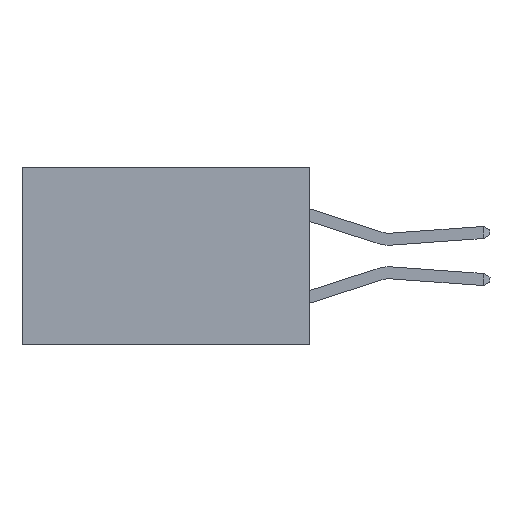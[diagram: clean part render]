
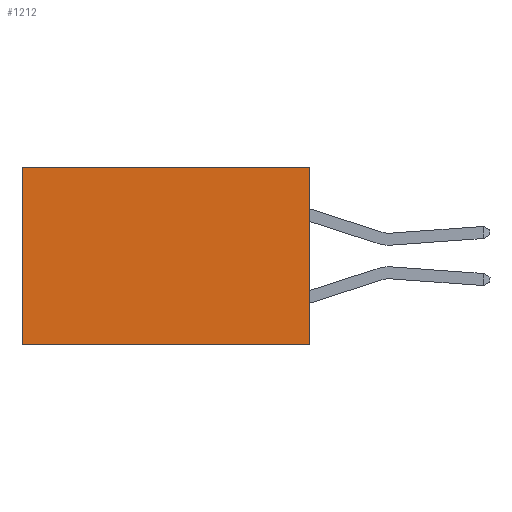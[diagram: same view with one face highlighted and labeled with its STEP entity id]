
A CAD part, left-side view. The second image highlights one B-rep face of the part: STEP entity #1212.
In plain terms, the highlighted planar face has unit normal (-1, 0, 0).
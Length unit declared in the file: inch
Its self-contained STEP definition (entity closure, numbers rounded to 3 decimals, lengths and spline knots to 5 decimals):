
#416 = EDGE_CURVE ( 'NONE', #12604, #13250, #8618, .T. ) ;
#594 = LINE ( 'NONE', #6916, #5492 ) ;
#1009 = DIRECTION ( 'NONE',  ( 0., 1., 0. ) ) ;
#1035 = ORIENTED_EDGE ( 'NONE', *, *, #416, .T. ) ;
#1129 = CARTESIAN_POINT ( 'NONE',  ( 0.298, 0., 0. ) ) ;
#1212 = ADVANCED_FACE ( 'NONE', ( #10508 ), #1586, .F. ) ;
#1256 = EDGE_LOOP ( 'NONE', ( #1035, #4736, #8461, #6330 ) ) ;
#1586 = PLANE ( 'NONE',  #8100 ) ;
#1635 = DIRECTION ( 'NONE',  ( 1., 0., 0. ) ) ;
#2235 = EDGE_CURVE ( 'NONE', #8248, #12604, #14859, .T. ) ;
#2613 = VECTOR ( 'NONE', #8156, 39.37008 ) ;
#4736 = ORIENTED_EDGE ( 'NONE', *, *, #14044, .F. ) ;
#4830 = VERTEX_POINT ( 'NONE', #8062 ) ;
#5492 = VECTOR ( 'NONE', #9350, 39.37008 ) ;
#5828 = CARTESIAN_POINT ( 'NONE',  ( 0.298, 0.6, 0. ) ) ;
#6102 = CARTESIAN_POINT ( 'NONE',  ( 0.298, 0.6, -0.37 ) ) ;
#6330 = ORIENTED_EDGE ( 'NONE', *, *, #2235, .T. ) ;
#6556 = DIRECTION ( 'NONE',  ( 0., 0., -1. ) ) ;
#6916 = CARTESIAN_POINT ( 'NONE',  ( 0.298, 0., -0.37 ) ) ;
#7901 = LINE ( 'NONE', #9403, #13182 ) ;
#8062 = CARTESIAN_POINT ( 'NONE',  ( 0.298, 0., -0.37 ) ) ;
#8100 = AXIS2_PLACEMENT_3D ( 'NONE', #15417, #1635, #6556 ) ;
#8156 = DIRECTION ( 'NONE',  ( 0., 0., -1. ) ) ;
#8248 = VERTEX_POINT ( 'NONE', #15392 ) ;
#8461 = ORIENTED_EDGE ( 'NONE', *, *, #12594, .F. ) ;
#8618 = LINE ( 'NONE', #5828, #2613 ) ;
#9350 = DIRECTION ( 'NONE',  ( 0., 1., 0. ) ) ;
#9403 = CARTESIAN_POINT ( 'NONE',  ( 0.298, 0., 0. ) ) ;
#10508 = FACE_OUTER_BOUND ( 'NONE', #1256, .T. ) ;
#10814 = DIRECTION ( 'NONE',  ( 0., 0., -1. ) ) ;
#12594 = EDGE_CURVE ( 'NONE', #8248, #4830, #7901, .T. ) ;
#12604 = VERTEX_POINT ( 'NONE', #15854 ) ;
#13060 = VECTOR ( 'NONE', #1009, 39.37008 ) ;
#13182 = VECTOR ( 'NONE', #10814, 39.37008 ) ;
#13250 = VERTEX_POINT ( 'NONE', #6102 ) ;
#14044 = EDGE_CURVE ( 'NONE', #4830, #13250, #594, .T. ) ;
#14859 = LINE ( 'NONE', #1129, #13060 ) ;
#15392 = CARTESIAN_POINT ( 'NONE',  ( 0.298, 0., 0. ) ) ;
#15417 = CARTESIAN_POINT ( 'NONE',  ( 0.298, 0., 0. ) ) ;
#15854 = CARTESIAN_POINT ( 'NONE',  ( 0.298, 0.6, 0. ) ) ;
